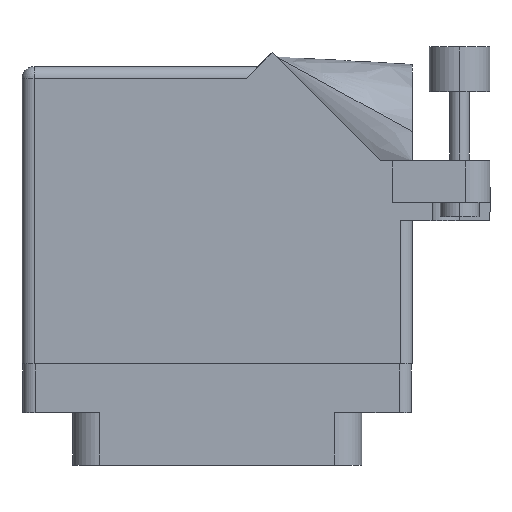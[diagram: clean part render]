
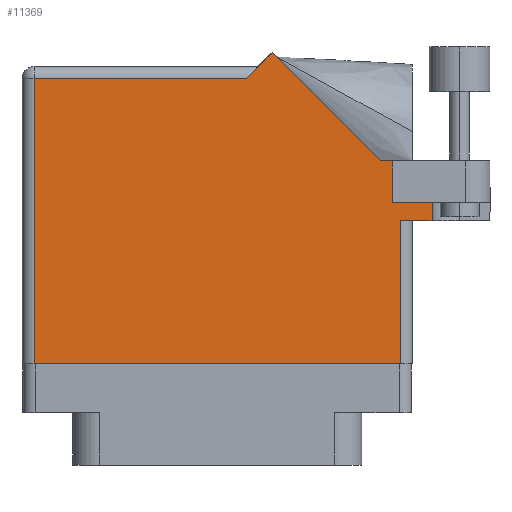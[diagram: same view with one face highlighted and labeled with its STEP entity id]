
A CAD part, front view. The second image highlights one B-rep face of the part: STEP entity #11369.
In plain terms, the highlighted face is planar.
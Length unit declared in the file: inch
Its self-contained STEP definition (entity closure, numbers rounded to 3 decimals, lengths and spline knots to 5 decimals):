
#135 = ORIENTED_EDGE ( 'NONE', *, *, #35602, .T. ) ;
#845 = PLANE ( 'NONE',  #31894 ) ;
#973 = VECTOR ( 'NONE', #10021, 39.37008 ) ;
#1683 = DIRECTION ( 'NONE',  ( 1., 0., 0. ) ) ;
#1969 = VECTOR ( 'NONE', #22462, 39.37008 ) ;
#2517 = CARTESIAN_POINT ( 'NONE',  ( -1.005, -0.1, 0.455 ) ) ;
#2745 = LINE ( 'NONE', #35493, #973 ) ;
#3022 = CARTESIAN_POINT ( 'NONE',  ( 1.405, 0.944, 0.455 ) ) ;
#3899 = CARTESIAN_POINT ( 'NONE',  ( -1.005, 1.368, 0.455 ) ) ;
#4778 = ORIENTED_EDGE ( 'NONE', *, *, #13859, .T. ) ;
#4892 = VERTEX_POINT ( 'NONE', #21278 ) ;
#5161 = ORIENTED_EDGE ( 'NONE', *, *, #19950, .T. ) ;
#5196 = LINE ( 'NONE', #29033, #9558 ) ;
#5924 = ORIENTED_EDGE ( 'NONE', *, *, #29139, .T. ) ;
#6462 = ORIENTED_EDGE ( 'NONE', *, *, #12276, .F. ) ;
#6815 = VERTEX_POINT ( 'NONE', #8198 ) ;
#7339 = CARTESIAN_POINT ( 'NONE',  ( 1.1065, 0.637, 0.455 ) ) ;
#7848 = EDGE_CURVE ( 'NONE', #4892, #10126, #20896, .T. ) ;
#8198 = CARTESIAN_POINT ( 'NONE',  ( 0.15, 1.368, 0.455 ) ) ;
#9558 = VECTOR ( 'NONE', #34833, 39.37008 ) ;
#9597 = VERTEX_POINT ( 'NONE', #34291 ) ;
#10021 = DIRECTION ( 'NONE',  ( 0., -1., 0. ) ) ;
#10126 = VERTEX_POINT ( 'NONE', #12313 ) ;
#10476 = EDGE_CURVE ( 'NONE', #10126, #29824, #23145, .T. ) ;
#10911 = EDGE_CURVE ( 'NONE', #23367, #23510, #5196, .T. ) ;
#11025 = EDGE_CURVE ( 'NONE', #9597, #13136, #32756, .T. ) ;
#11369 = ADVANCED_FACE ( 'NONE', ( #13410 ), #845, .F. ) ;
#11516 = LINE ( 'NONE', #2517, #24223 ) ;
#11597 = CARTESIAN_POINT ( 'NONE',  ( 0.943, 0.637, 0.455 ) ) ;
#12276 = EDGE_CURVE ( 'NONE', #13136, #29824, #2745, .T. ) ;
#12313 = CARTESIAN_POINT ( 'NONE',  ( 0.943, 0.637, 0.455 ) ) ;
#12636 = CARTESIAN_POINT ( 'NONE',  ( 0.83942, 0.944, 0.455 ) ) ;
#13136 = VERTEX_POINT ( 'NONE', #20817 ) ;
#13410 = FACE_OUTER_BOUND ( 'NONE', #21054, .T. ) ;
#13445 = VECTOR ( 'NONE', #25631, 39.37008 ) ;
#13859 = EDGE_CURVE ( 'NONE', #23510, #4892, #11516, .T. ) ;
#13890 = DIRECTION ( 'NONE',  ( -1., 0., 0. ) ) ;
#14279 = VECTOR ( 'NONE', #17946, 39.37008 ) ;
#14749 = CARTESIAN_POINT ( 'NONE',  ( 0.905, 0.731, 0.455 ) ) ;
#15042 = DIRECTION ( 'NONE',  ( -1., 0., 0. ) ) ;
#15678 = ORIENTED_EDGE ( 'NONE', *, *, #21696, .T. ) ;
#15715 = VECTOR ( 'NONE', #23304, 39.37008 ) ;
#16080 = LINE ( 'NONE', #12636, #14279 ) ;
#16136 = DIRECTION ( 'NONE',  ( 1., 0., 0. ) ) ;
#16372 = CARTESIAN_POINT ( 'NONE',  ( 0.905, 0.731, 0.455 ) ) ;
#16420 = VERTEX_POINT ( 'NONE', #27544 ) ;
#16992 = CARTESIAN_POINT ( 'NONE',  ( 0.212, 1.43, 0.455 ) ) ;
#17946 = DIRECTION ( 'NONE',  ( -0.707, 0.707, 0. ) ) ;
#18616 = LINE ( 'NONE', #16992, #1969 ) ;
#19950 = EDGE_CURVE ( 'NONE', #9597, #34721, #20112, .T. ) ;
#20112 = LINE ( 'NONE', #16372, #26649 ) ;
#20817 = CARTESIAN_POINT ( 'NONE',  ( 1.1065, 0.731, 0.455 ) ) ;
#20893 = VECTOR ( 'NONE', #15042, 39.37008 ) ;
#20896 = LINE ( 'NONE', #11597, #13445 ) ;
#21054 = EDGE_LOOP ( 'NONE', ( #4778, #23971, #22277, #6462, #31162, #5161, #5924, #15678, #135, #26668, #29529 ) ) ;
#21278 = CARTESIAN_POINT ( 'NONE',  ( 0.943, -0.1, 0.455 ) ) ;
#21696 = EDGE_CURVE ( 'NONE', #26494, #16420, #16080, .T. ) ;
#22277 = ORIENTED_EDGE ( 'NONE', *, *, #10476, .T. ) ;
#22324 = DIRECTION ( 'NONE',  ( 0., 1., 0. ) ) ;
#22462 = DIRECTION ( 'NONE',  ( -0.707, -0.707, 0. ) ) ;
#23145 = LINE ( 'NONE', #32287, #35010 ) ;
#23304 = DIRECTION ( 'NONE',  ( 1., 0., 0. ) ) ;
#23367 = VERTEX_POINT ( 'NONE', #25173 ) ;
#23510 = VERTEX_POINT ( 'NONE', #26615 ) ;
#23971 = ORIENTED_EDGE ( 'NONE', *, *, #7848, .T. ) ;
#24223 = VECTOR ( 'NONE', #16136, 39.37008 ) ;
#25173 = CARTESIAN_POINT ( 'NONE',  ( -0.943, 1.368, 0.455 ) ) ;
#25631 = DIRECTION ( 'NONE',  ( 0., 1., 0. ) ) ;
#26025 = CARTESIAN_POINT ( 'NONE',  ( -1.005, 1.43, 0.455 ) ) ;
#26148 = DIRECTION ( 'NONE',  ( 0., 0., -1. ) ) ;
#26494 = VERTEX_POINT ( 'NONE', #29648 ) ;
#26615 = CARTESIAN_POINT ( 'NONE',  ( -0.943, -0.1, 0.455 ) ) ;
#26649 = VECTOR ( 'NONE', #22324, 39.37008 ) ;
#26668 = ORIENTED_EDGE ( 'NONE', *, *, #34426, .T. ) ;
#27544 = CARTESIAN_POINT ( 'NONE',  ( 0.28271, 1.50071, 0.455 ) ) ;
#28043 = CARTESIAN_POINT ( 'NONE',  ( 0.905, 0.944, 0.455 ) ) ;
#28686 = VECTOR ( 'NONE', #13890, 39.37008 ) ;
#29033 = CARTESIAN_POINT ( 'NONE',  ( -0.943, -0.1, 0.455 ) ) ;
#29139 = EDGE_CURVE ( 'NONE', #34721, #26494, #36237, .T. ) ;
#29529 = ORIENTED_EDGE ( 'NONE', *, *, #10911, .T. ) ;
#29648 = CARTESIAN_POINT ( 'NONE',  ( 0.83942, 0.944, 0.455 ) ) ;
#29824 = VERTEX_POINT ( 'NONE', #7339 ) ;
#31162 = ORIENTED_EDGE ( 'NONE', *, *, #11025, .F. ) ;
#31894 = AXIS2_PLACEMENT_3D ( 'NONE', #26025, #26148, #34526 ) ;
#32287 = CARTESIAN_POINT ( 'NONE',  ( 1.005, 0.637, 0.455 ) ) ;
#32756 = LINE ( 'NONE', #14749, #15715 ) ;
#33177 = LINE ( 'NONE', #3899, #20893 ) ;
#34291 = CARTESIAN_POINT ( 'NONE',  ( 0.905, 0.731, 0.455 ) ) ;
#34426 = EDGE_CURVE ( 'NONE', #6815, #23367, #33177, .T. ) ;
#34526 = DIRECTION ( 'NONE',  ( -1., 0., 0. ) ) ;
#34721 = VERTEX_POINT ( 'NONE', #28043 ) ;
#34833 = DIRECTION ( 'NONE',  ( 0., -1., 0. ) ) ;
#35010 = VECTOR ( 'NONE', #1683, 39.37008 ) ;
#35493 = CARTESIAN_POINT ( 'NONE',  ( 1.1065, 1.06177, 0.455 ) ) ;
#35602 = EDGE_CURVE ( 'NONE', #16420, #6815, #18616, .T. ) ;
#36237 = LINE ( 'NONE', #3022, #28686 ) ;
